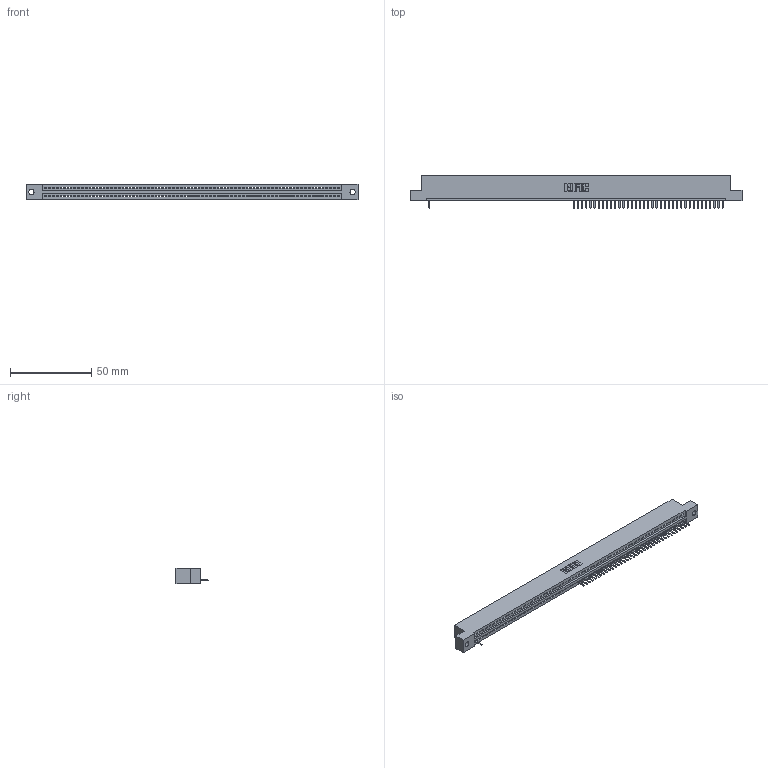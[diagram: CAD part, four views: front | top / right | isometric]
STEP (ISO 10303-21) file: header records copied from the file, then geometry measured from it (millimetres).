
FILE_DESCRIPTION (( 'STEP AP203' ), '1' );
FILE_NAME ('395-072-520-102.STEP', '2018-11-27T07:47:12', ( '' ), ( '' ), 'SwSTEP 2.0', 'SolidWorks 2016', '' );
FILE_SCHEMA (( 'CONFIG_CONTROL_DESIGN' ));
Length unit declared in the file: inch
Products named in the file (3): 345 Part_Flush Mounting Lugs - 0.128 Dia; 395-072-520-102; 345-292-001_345-293-120
Assembly tree (39 placements, depth 2):
  395-072-520-102
    345 Part_Flush Mounting Lugs - 0.128 Dia
    345-292-001_345-293-120  x38
Bounding box: 204.09 x 19.68 x 9.4 mm (x, y, z)
Volume: 19095 mm3; surface area: 23086.6 mm2
Topology: 39 solids, 39 shells, 3026 faces, 9169 edges, 6010 vertices
Faces by surface type: plane 2152, cylinder 874
Entity records: 49179 total; most frequent: ORIENTED_EDGE 8718, CARTESIAN_POINT 8690, DIRECTION 7495, EDGE_CURVE 4359, VECTOR 3935, LINE 3935, VERTEX_POINT 2902, AXIS2_PLACEMENT_3D 1780
